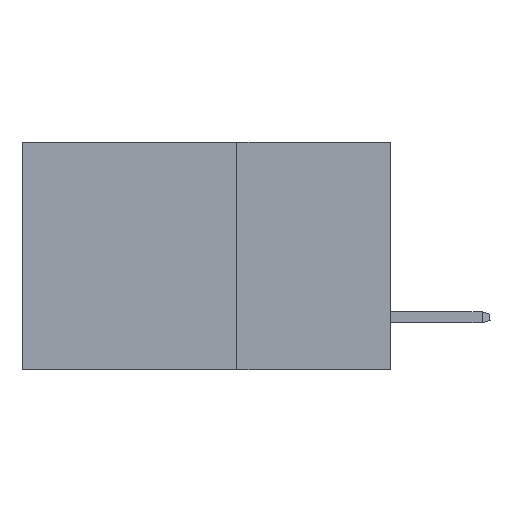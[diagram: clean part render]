
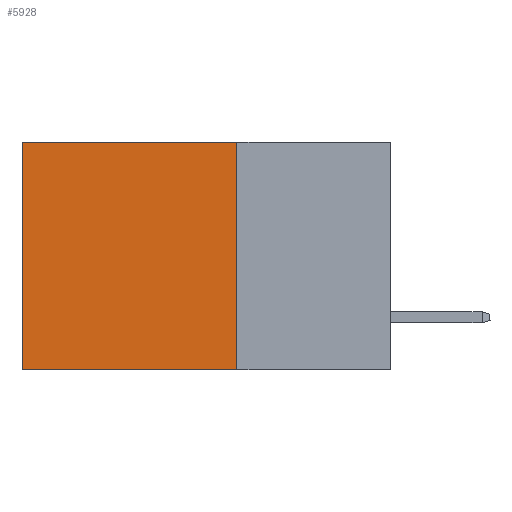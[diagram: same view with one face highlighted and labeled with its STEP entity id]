
A CAD part, left-side view. The second image highlights one B-rep face of the part: STEP entity #5928.
In plain terms, the highlighted planar face has unit normal (-1, 0, 0).
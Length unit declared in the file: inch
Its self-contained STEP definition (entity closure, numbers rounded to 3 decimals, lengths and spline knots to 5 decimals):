
#381 = VERTEX_POINT ( 'NONE', #18024 ) ;
#1350 = DIRECTION ( 'NONE',  ( 0., 0., -1. ) ) ;
#3315 = AXIS2_PLACEMENT_3D ( 'NONE', #30822, #23403, #1350 ) ;
#5539 = VERTEX_POINT ( 'NONE', #26950 ) ;
#5928 = ADVANCED_FACE ( 'NONE', ( #46209 ), #42938, .F. ) ;
#6936 = LINE ( 'NONE', #42752, #24776 ) ;
#7483 = EDGE_CURVE ( 'NONE', #381, #5539, #15536, .T. ) ;
#8319 = ORIENTED_EDGE ( 'NONE', *, *, #7483, .F. ) ;
#10051 = CARTESIAN_POINT ( 'NONE',  ( 0.2875, 0.6, 0. ) ) ;
#13250 = VECTOR ( 'NONE', #31572, 39.37008 ) ;
#15536 = LINE ( 'NONE', #42551, #13250 ) ;
#15918 = CARTESIAN_POINT ( 'NONE',  ( 0.2875, 0.6, 0. ) ) ;
#18024 = CARTESIAN_POINT ( 'NONE',  ( 0.2875, 0.25, -0.37 ) ) ;
#22636 = CARTESIAN_POINT ( 'NONE',  ( 0.2875, 0.25, 0. ) ) ;
#23403 = DIRECTION ( 'NONE',  ( 1., 0., 0. ) ) ;
#23591 = VERTEX_POINT ( 'NONE', #15918 ) ;
#23867 = EDGE_CURVE ( 'NONE', #23591, #5539, #28634, .T. ) ;
#24776 = VECTOR ( 'NONE', #32083, 39.37008 ) ;
#25040 = DIRECTION ( 'NONE',  ( 0., 0., -1. ) ) ;
#26650 = DIRECTION ( 'NONE',  ( 0., 1., 0. ) ) ;
#26950 = CARTESIAN_POINT ( 'NONE',  ( 0.2875, 0.6, -0.37 ) ) ;
#27051 = EDGE_CURVE ( 'NONE', #35927, #381, #6936, .T. ) ;
#28119 = ORIENTED_EDGE ( 'NONE', *, *, #42064, .T. ) ;
#28634 = LINE ( 'NONE', #10051, #43073 ) ;
#29990 = EDGE_LOOP ( 'NONE', ( #37548, #8319, #45377, #28119 ) ) ;
#30822 = CARTESIAN_POINT ( 'NONE',  ( 0.2875, 0.25, 0. ) ) ;
#31572 = DIRECTION ( 'NONE',  ( 0., 1., 0. ) ) ;
#31963 = CARTESIAN_POINT ( 'NONE',  ( 0.2875, 0.25, 0. ) ) ;
#32083 = DIRECTION ( 'NONE',  ( 0., 0., -1. ) ) ;
#32400 = VECTOR ( 'NONE', #26650, 39.37008 ) ;
#35927 = VERTEX_POINT ( 'NONE', #31963 ) ;
#37548 = ORIENTED_EDGE ( 'NONE', *, *, #23867, .T. ) ;
#41117 = LINE ( 'NONE', #22636, #32400 ) ;
#42064 = EDGE_CURVE ( 'NONE', #35927, #23591, #41117, .T. ) ;
#42551 = CARTESIAN_POINT ( 'NONE',  ( 0.2875, 0.25, -0.37 ) ) ;
#42752 = CARTESIAN_POINT ( 'NONE',  ( 0.2875, 0.25, 0. ) ) ;
#42938 = PLANE ( 'NONE',  #3315 ) ;
#43073 = VECTOR ( 'NONE', #25040, 39.37008 ) ;
#45377 = ORIENTED_EDGE ( 'NONE', *, *, #27051, .F. ) ;
#46209 = FACE_OUTER_BOUND ( 'NONE', #29990, .T. ) ;
